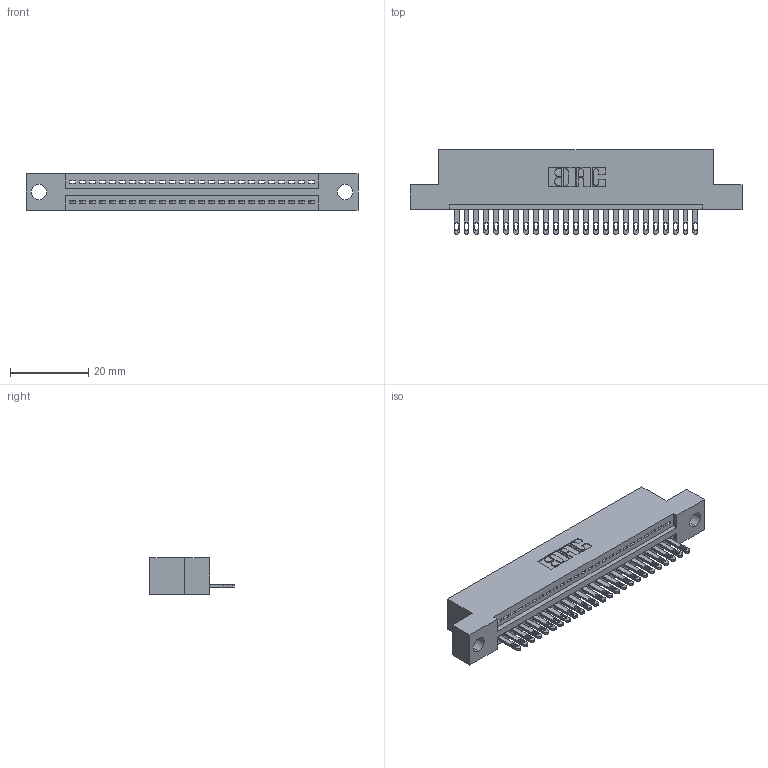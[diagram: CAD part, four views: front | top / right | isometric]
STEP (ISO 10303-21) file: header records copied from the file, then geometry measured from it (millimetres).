
FILE_DESCRIPTION (( 'STEP AP203' ), '1' );
FILE_NAME ('345-025-500-104.STEP', '2021-05-26T14:28:54', ( '' ), ( '' ), 'SwSTEP 2.0', 'SolidWorks 2020', '' );
FILE_SCHEMA (( 'CONFIG_CONTROL_DESIGN' ));
Length unit declared in the file: inch
Products named in the file (3): 345-292-001_345-293-100; 345-025-500-104; 345 Part_Flush Mounting Lugs - 0.156 Dia-TI
Assembly tree (26 placements, depth 2):
  345-025-500-104
    345 Part_Flush Mounting Lugs - 0.156 Dia-TI
    345-292-001_345-293-100  x25
Bounding box: 84.71 x 21.51 x 9.4 mm (x, y, z)
Volume: 7816 mm3; surface area: 10054.3 mm2
Topology: 26 solids, 26 shells, 1490 faces, 4577 edges, 3050 vertices
Faces by surface type: plane 944, cylinder 546
Entity records: 21453 total; most frequent: CARTESIAN_POINT 3725, ORIENTED_EDGE 3682, DIRECTION 3279, EDGE_CURVE 1841, LINE 1605, VECTOR 1605, VERTEX_POINT 1226, AXIS2_PLACEMENT_3D 837
